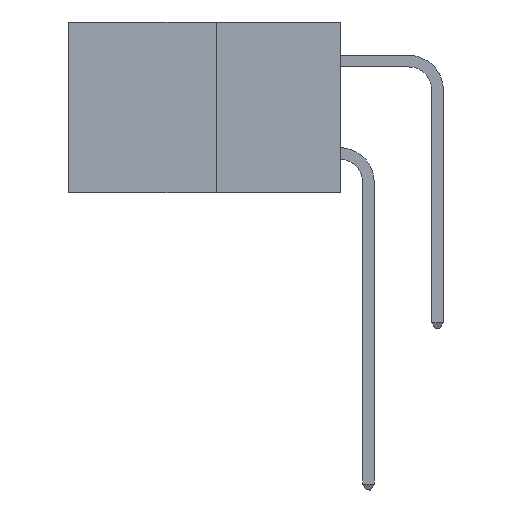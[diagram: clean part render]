
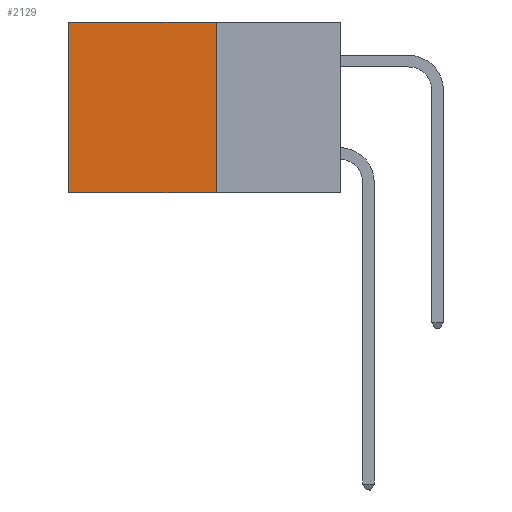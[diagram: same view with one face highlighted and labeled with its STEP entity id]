
A CAD part, left-side view. The second image highlights one B-rep face of the part: STEP entity #2129.
In plain terms, the highlighted planar face has unit normal (-1, 0, 0).
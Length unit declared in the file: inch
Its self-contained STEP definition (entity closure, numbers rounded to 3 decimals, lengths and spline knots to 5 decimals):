
#1332 = VECTOR ( 'NONE', #8287, 39.37008 ) ;
#1588 = CARTESIAN_POINT ( 'NONE',  ( 0.277, 0.27, -0.37 ) ) ;
#1608 = LINE ( 'NONE', #1588, #7764 ) ;
#1612 = EDGE_CURVE ( 'NONE', #4520, #6506, #9311, .T. ) ;
#1673 = VECTOR ( 'NONE', #6944, 39.37008 ) ;
#1790 = VERTEX_POINT ( 'NONE', #5192 ) ;
#2129 = ADVANCED_FACE ( 'NONE', ( #2444 ), #5731, .F. ) ;
#2166 = AXIS2_PLACEMENT_3D ( 'NONE', #3413, #9325, #3283 ) ;
#2409 = DIRECTION ( 'NONE',  ( 0., 0., -1. ) ) ;
#2444 = FACE_OUTER_BOUND ( 'NONE', #3074, .T. ) ;
#2658 = ORIENTED_EDGE ( 'NONE', *, *, #7037, .T. ) ;
#2713 = CARTESIAN_POINT ( 'NONE',  ( 0.277, 0.27, 0. ) ) ;
#3074 = EDGE_LOOP ( 'NONE', ( #5406, #9446, #6191, #2658 ) ) ;
#3283 = DIRECTION ( 'NONE',  ( 0., 0., -1. ) ) ;
#3413 = CARTESIAN_POINT ( 'NONE',  ( 0.277, 0.27, -0.37 ) ) ;
#3423 = EDGE_CURVE ( 'NONE', #8564, #6506, #4315, .T. ) ;
#3469 = VECTOR ( 'NONE', #10316, 39.37008 ) ;
#4297 = CARTESIAN_POINT ( 'NONE',  ( 0.277, 0.27, -0.37 ) ) ;
#4315 = LINE ( 'NONE', #5156, #1673 ) ;
#4520 = VERTEX_POINT ( 'NONE', #7380 ) ;
#4598 = CARTESIAN_POINT ( 'NONE',  ( 0.277, 0.59, 0. ) ) ;
#5156 = CARTESIAN_POINT ( 'NONE',  ( 0.277, 0.59, -0.37 ) ) ;
#5192 = CARTESIAN_POINT ( 'NONE',  ( 0.277, 0.27, 0. ) ) ;
#5406 = ORIENTED_EDGE ( 'NONE', *, *, #3423, .T. ) ;
#5731 = PLANE ( 'NONE',  #2166 ) ;
#5877 = LINE ( 'NONE', #2713, #1332 ) ;
#6146 = EDGE_CURVE ( 'NONE', #1790, #4520, #1608, .T. ) ;
#6191 = ORIENTED_EDGE ( 'NONE', *, *, #6146, .F. ) ;
#6506 = VERTEX_POINT ( 'NONE', #6841 ) ;
#6841 = CARTESIAN_POINT ( 'NONE',  ( 0.277, 0.59, -0.37 ) ) ;
#6944 = DIRECTION ( 'NONE',  ( 0., 0., -1. ) ) ;
#7037 = EDGE_CURVE ( 'NONE', #1790, #8564, #5877, .T. ) ;
#7380 = CARTESIAN_POINT ( 'NONE',  ( 0.277, 0.27, -0.37 ) ) ;
#7764 = VECTOR ( 'NONE', #2409, 39.37008 ) ;
#8287 = DIRECTION ( 'NONE',  ( 0., 1., 0. ) ) ;
#8564 = VERTEX_POINT ( 'NONE', #4598 ) ;
#9311 = LINE ( 'NONE', #4297, #3469 ) ;
#9325 = DIRECTION ( 'NONE',  ( 1., 0., 0. ) ) ;
#9446 = ORIENTED_EDGE ( 'NONE', *, *, #1612, .F. ) ;
#10316 = DIRECTION ( 'NONE',  ( 0., 1., 0. ) ) ;
